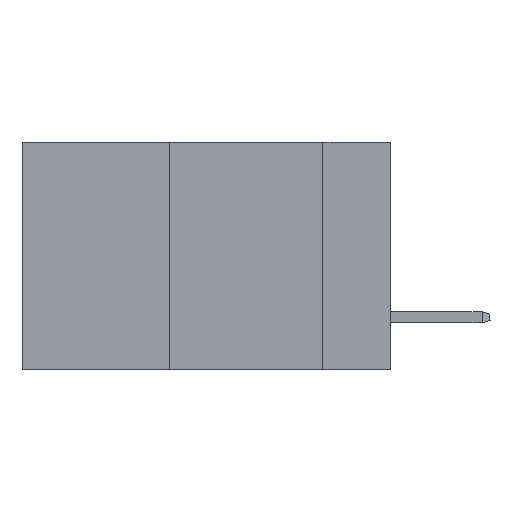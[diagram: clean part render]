
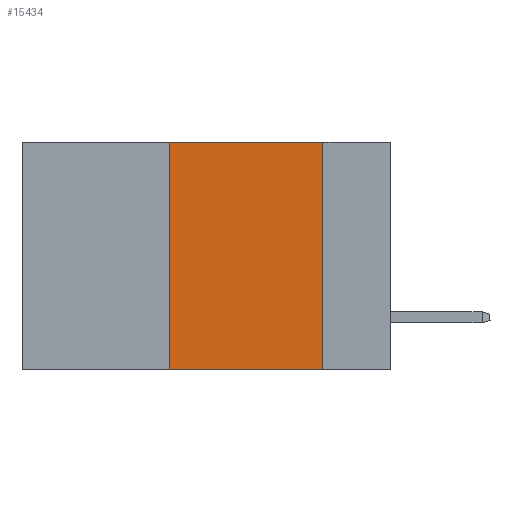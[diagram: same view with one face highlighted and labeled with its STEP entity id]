
A CAD part, left-side view. The second image highlights one B-rep face of the part: STEP entity #15434.
In plain terms, the highlighted planar face has unit normal (-1, 0, 0).
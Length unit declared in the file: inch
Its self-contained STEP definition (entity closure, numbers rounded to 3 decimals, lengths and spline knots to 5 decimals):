
#211 = CARTESIAN_POINT ( 'NONE',  ( 0., 0.11, 0. ) ) ;
#634 = AXIS2_PLACEMENT_3D ( 'NONE', #24287, #15028, #3692 ) ;
#1865 = DIRECTION ( 'NONE',  ( 0., 0., -1. ) ) ;
#2548 = CARTESIAN_POINT ( 'NONE',  ( 0., 0.6, 0. ) ) ;
#3045 = VECTOR ( 'NONE', #1865, 39.37008 ) ;
#3513 = VERTEX_POINT ( 'NONE', #211 ) ;
#3692 = DIRECTION ( 'NONE',  ( 0., 0., -1. ) ) ;
#4084 = EDGE_CURVE ( 'NONE', #7668, #12784, #21419, .T. ) ;
#4968 = CARTESIAN_POINT ( 'NONE',  ( 0., 0.36, -0.37 ) ) ;
#5368 = EDGE_CURVE ( 'NONE', #7668, #5804, #21924, .T. ) ;
#5505 = DIRECTION ( 'NONE',  ( 0., -1., 0. ) ) ;
#5612 = CARTESIAN_POINT ( 'NONE',  ( 0., 0.36, 0. ) ) ;
#5804 = VERTEX_POINT ( 'NONE', #10395 ) ;
#6442 = VECTOR ( 'NONE', #5505, 39.37008 ) ;
#6635 = EDGE_CURVE ( 'NONE', #3513, #12784, #13681, .T. ) ;
#7487 = ORIENTED_EDGE ( 'NONE', *, *, #17881, .F. ) ;
#7668 = VERTEX_POINT ( 'NONE', #4968 ) ;
#10395 = CARTESIAN_POINT ( 'NONE',  ( 0., 0.36, 0. ) ) ;
#11323 = ORIENTED_EDGE ( 'NONE', *, *, #6635, .F. ) ;
#11871 = DIRECTION ( 'NONE',  ( 0., -1., 0. ) ) ;
#12603 = CARTESIAN_POINT ( 'NONE',  ( 0., 0.11, -0.37 ) ) ;
#12784 = VERTEX_POINT ( 'NONE', #12603 ) ;
#12989 = VECTOR ( 'NONE', #11871, 39.37008 ) ;
#13187 = CARTESIAN_POINT ( 'NONE',  ( 0., 0.11, 0. ) ) ;
#13681 = LINE ( 'NONE', #13187, #3045 ) ;
#15028 = DIRECTION ( 'NONE',  ( 1., 0., 0. ) ) ;
#15434 = ADVANCED_FACE ( 'NONE', ( #19575 ), #20568, .F. ) ;
#17547 = ORIENTED_EDGE ( 'NONE', *, *, #5368, .F. ) ;
#17594 = VECTOR ( 'NONE', #18781, 39.37008 ) ;
#17881 = EDGE_CURVE ( 'NONE', #5804, #3513, #18565, .T. ) ;
#18118 = ORIENTED_EDGE ( 'NONE', *, *, #4084, .T. ) ;
#18565 = LINE ( 'NONE', #2548, #12989 ) ;
#18685 = CARTESIAN_POINT ( 'NONE',  ( 0., 0.6, -0.37 ) ) ;
#18781 = DIRECTION ( 'NONE',  ( 0., 0., 1. ) ) ;
#19575 = FACE_OUTER_BOUND ( 'NONE', #24051, .T. ) ;
#20568 = PLANE ( 'NONE',  #634 ) ;
#21419 = LINE ( 'NONE', #18685, #6442 ) ;
#21924 = LINE ( 'NONE', #5612, #17594 ) ;
#24051 = EDGE_LOOP ( 'NONE', ( #11323, #7487, #17547, #18118 ) ) ;
#24287 = CARTESIAN_POINT ( 'NONE',  ( 0., 0.6, 0. ) ) ;
